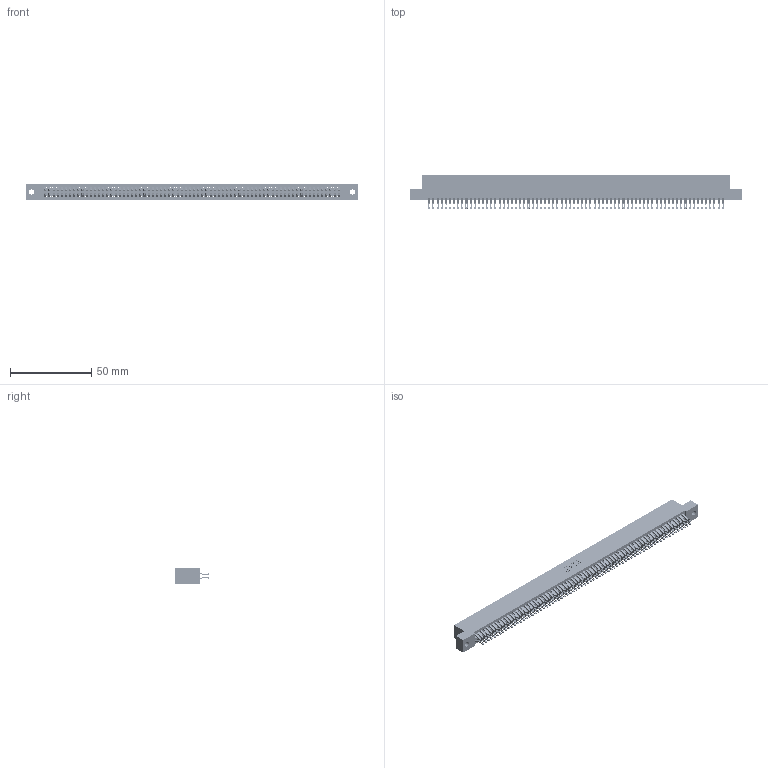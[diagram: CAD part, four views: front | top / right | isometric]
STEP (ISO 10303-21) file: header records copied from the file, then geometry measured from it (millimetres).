
FILE_DESCRIPTION (( 'STEP AP203' ), '1' );
FILE_NAME ('395-144-555-202.STEP', '2019-10-30T16:24:47', ( '' ), ( '' ), 'SwSTEP 2.0', 'SolidWorks 2016', '' );
FILE_SCHEMA (( 'CONFIG_CONTROL_DESIGN' ));
Length unit declared in the file: inch
Products named in the file (3): 395-144-555-202; 345 Part_Flush Mounting Lugs - 0.128 Dia; 345-292-001_555 Tail
Assembly tree (145 placements, depth 2):
  395-144-555-202
    345 Part_Flush Mounting Lugs - 0.128 Dia
    345-292-001_555 Tail  x144
Bounding box: 204.09 x 21.13 x 9.4 mm (x, y, z)
Volume: 20484.9 mm3; surface area: 32041.1 mm2
Topology: 145 solids, 145 shells, 8190 faces, 25829 edges, 17218 vertices
Faces by surface type: plane 4544, cylinder 3646
Entity records: 52783 total; most frequent: CARTESIAN_POINT 8854, ORIENTED_EDGE 8758, DIRECTION 7739, EDGE_CURVE 4379, VECTOR 3939, LINE 3939, VERTEX_POINT 2918, AXIS2_PLACEMENT_3D 1900
